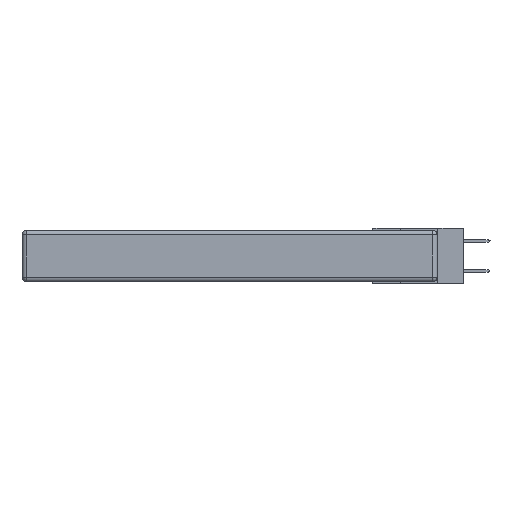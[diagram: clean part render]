
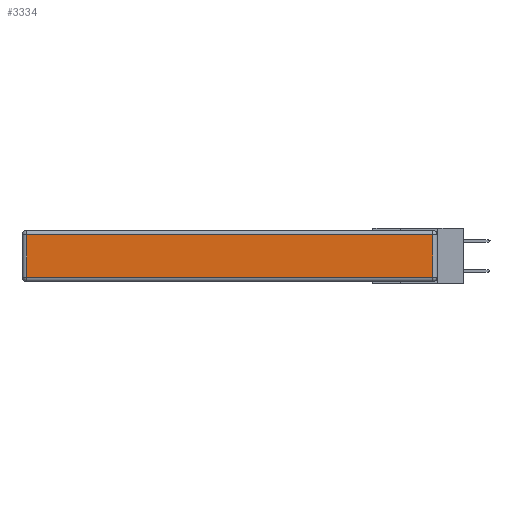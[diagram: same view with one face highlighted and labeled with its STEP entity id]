
A CAD part, left-side view. The second image highlights one B-rep face of the part: STEP entity #3334.
In plain terms, the highlighted planar face has unit normal (-1, 0, 0).
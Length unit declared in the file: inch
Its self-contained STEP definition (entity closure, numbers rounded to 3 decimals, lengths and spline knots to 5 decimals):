
#97 = CARTESIAN_POINT ( 'NONE',  ( 0., 0.03, -0.343 ) ) ;
#125 = ORIENTED_EDGE ( 'NONE', *, *, #9798, .T. ) ;
#191 = VECTOR ( 'NONE', #3180, 39.37008 ) ;
#439 = CARTESIAN_POINT ( 'NONE',  ( 0., 2.72, -0.03 ) ) ;
#1019 = CARTESIAN_POINT ( 'NONE',  ( 0., 0.03, -0.313 ) ) ;
#1320 = EDGE_CURVE ( 'NONE', #25941, #8813, #25487, .T. ) ;
#1384 = ORIENTED_EDGE ( 'NONE', *, *, #6078, .T. ) ;
#2423 = EDGE_CURVE ( 'NONE', #2735, #25941, #3286, .T. ) ;
#2735 = VERTEX_POINT ( 'NONE', #9352 ) ;
#3180 = DIRECTION ( 'NONE',  ( 0., 0., -1. ) ) ;
#3286 = LINE ( 'NONE', #7607, #16100 ) ;
#3334 = ADVANCED_FACE ( 'NONE', ( #8078 ), #21851, .T. ) ;
#3357 = ORIENTED_EDGE ( 'NONE', *, *, #1320, .T. ) ;
#3491 = ORIENTED_EDGE ( 'NONE', *, *, #2423, .T. ) ;
#4041 = DIRECTION ( 'NONE',  ( 0., -1., 0. ) ) ;
#4401 = VECTOR ( 'NONE', #4041, 39.37008 ) ;
#5456 = DIRECTION ( 'NONE',  ( -1., 0., 0. ) ) ;
#5550 = VECTOR ( 'NONE', #14744, 39.37008 ) ;
#6078 = EDGE_CURVE ( 'NONE', #8813, #19847, #14008, .T. ) ;
#7516 = CARTESIAN_POINT ( 'NONE',  ( 0., 2.72, -0.343 ) ) ;
#7607 = CARTESIAN_POINT ( 'NONE',  ( 0., 2.75, -0.03 ) ) ;
#8078 = FACE_OUTER_BOUND ( 'NONE', #13234, .T. ) ;
#8813 = VERTEX_POINT ( 'NONE', #19708 ) ;
#9352 = CARTESIAN_POINT ( 'NONE',  ( 0., 0.03, -0.03 ) ) ;
#9798 = EDGE_CURVE ( 'NONE', #19847, #2735, #15810, .T. ) ;
#11373 = DIRECTION ( 'NONE',  ( 0., 0., 1. ) ) ;
#11479 = DIRECTION ( 'NONE',  ( 0., 1., 0. ) ) ;
#13234 = EDGE_LOOP ( 'NONE', ( #1384, #125, #3491, #3357 ) ) ;
#14008 = LINE ( 'NONE', #24477, #4401 ) ;
#14744 = DIRECTION ( 'NONE',  ( 0., 0., 1. ) ) ;
#15810 = LINE ( 'NONE', #97, #5550 ) ;
#16100 = VECTOR ( 'NONE', #11479, 39.37008 ) ;
#19397 = AXIS2_PLACEMENT_3D ( 'NONE', #23649, #5456, #11373 ) ;
#19708 = CARTESIAN_POINT ( 'NONE',  ( 0., 2.72, -0.313 ) ) ;
#19847 = VERTEX_POINT ( 'NONE', #1019 ) ;
#21851 = PLANE ( 'NONE',  #19397 ) ;
#23649 = CARTESIAN_POINT ( 'NONE',  ( 0., 0., -0.343 ) ) ;
#24477 = CARTESIAN_POINT ( 'NONE',  ( 0., 0., -0.313 ) ) ;
#25487 = LINE ( 'NONE', #7516, #191 ) ;
#25941 = VERTEX_POINT ( 'NONE', #439 ) ;
